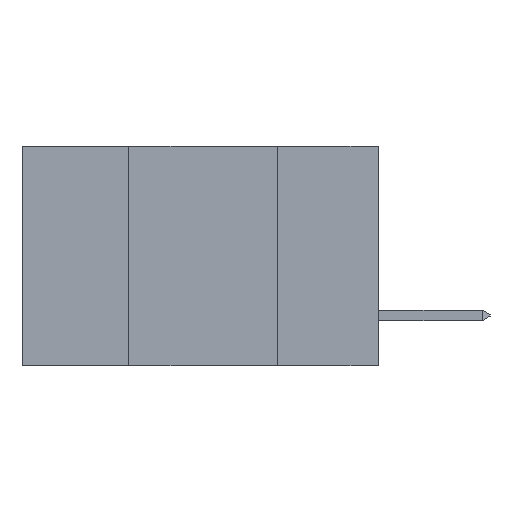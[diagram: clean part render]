
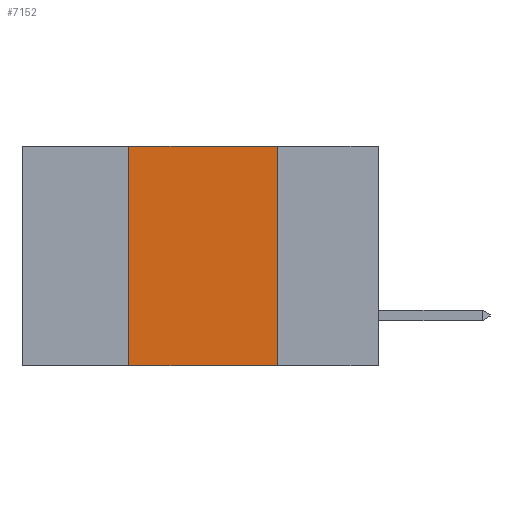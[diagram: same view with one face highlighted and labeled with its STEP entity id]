
A CAD part, left-side view. The second image highlights one B-rep face of the part: STEP entity #7152.
In plain terms, the highlighted planar face has unit normal (-1, 0, 0).
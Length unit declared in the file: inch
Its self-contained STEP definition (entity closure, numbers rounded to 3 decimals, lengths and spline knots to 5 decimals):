
#277 = VERTEX_POINT ( 'NONE', #20154 ) ;
#617 = LINE ( 'NONE', #13331, #17568 ) ;
#857 = CARTESIAN_POINT ( 'NONE',  ( 0., 0.17, 0. ) ) ;
#1165 = CARTESIAN_POINT ( 'NONE',  ( 0., 0.42, 0. ) ) ;
#1311 = EDGE_CURVE ( 'NONE', #20079, #12145, #8960, .T. ) ;
#2478 = EDGE_LOOP ( 'NONE', ( #3223, #17684, #10835, #9730 ) ) ;
#2823 = EDGE_CURVE ( 'NONE', #12145, #13385, #617, .T. ) ;
#3223 = ORIENTED_EDGE ( 'NONE', *, *, #2823, .F. ) ;
#3263 = CARTESIAN_POINT ( 'NONE',  ( 0., 0.42, 0. ) ) ;
#4253 = LINE ( 'NONE', #3263, #12891 ) ;
#6172 = EDGE_CURVE ( 'NONE', #277, #20079, #4253, .T. ) ;
#6789 = LINE ( 'NONE', #10701, #15380 ) ;
#7152 = ADVANCED_FACE ( 'NONE', ( #19433 ), #16741, .F. ) ;
#8960 = LINE ( 'NONE', #18336, #13566 ) ;
#9730 = ORIENTED_EDGE ( 'NONE', *, *, #16539, .T. ) ;
#10701 = CARTESIAN_POINT ( 'NONE',  ( 0., 0.6, -0.37 ) ) ;
#10835 = ORIENTED_EDGE ( 'NONE', *, *, #6172, .F. ) ;
#12145 = VERTEX_POINT ( 'NONE', #857 ) ;
#12398 = DIRECTION ( 'NONE',  ( 0., 0., 1. ) ) ;
#12891 = VECTOR ( 'NONE', #12398, 39.37008 ) ;
#13331 = CARTESIAN_POINT ( 'NONE',  ( 0., 0.17, 0. ) ) ;
#13385 = VERTEX_POINT ( 'NONE', #17845 ) ;
#13566 = VECTOR ( 'NONE', #20121, 39.37008 ) ;
#15380 = VECTOR ( 'NONE', #15734, 39.37008 ) ;
#15734 = DIRECTION ( 'NONE',  ( 0., -1., 0. ) ) ;
#16539 = EDGE_CURVE ( 'NONE', #277, #13385, #6789, .T. ) ;
#16741 = PLANE ( 'NONE',  #18127 ) ;
#17568 = VECTOR ( 'NONE', #20806, 39.37008 ) ;
#17684 = ORIENTED_EDGE ( 'NONE', *, *, #1311, .F. ) ;
#17742 = CARTESIAN_POINT ( 'NONE',  ( 0., 0.6, 0. ) ) ;
#17845 = CARTESIAN_POINT ( 'NONE',  ( 0., 0.17, -0.37 ) ) ;
#17976 = DIRECTION ( 'NONE',  ( 0., 0., -1. ) ) ;
#17983 = DIRECTION ( 'NONE',  ( 1., 0., 0. ) ) ;
#18127 = AXIS2_PLACEMENT_3D ( 'NONE', #17742, #17983, #17976 ) ;
#18336 = CARTESIAN_POINT ( 'NONE',  ( 0., 0.6, 0. ) ) ;
#19433 = FACE_OUTER_BOUND ( 'NONE', #2478, .T. ) ;
#20079 = VERTEX_POINT ( 'NONE', #1165 ) ;
#20121 = DIRECTION ( 'NONE',  ( 0., -1., 0. ) ) ;
#20154 = CARTESIAN_POINT ( 'NONE',  ( 0., 0.42, -0.37 ) ) ;
#20806 = DIRECTION ( 'NONE',  ( 0., 0., -1. ) ) ;
